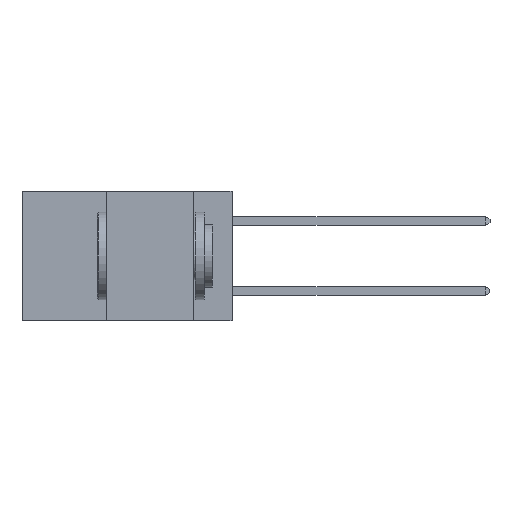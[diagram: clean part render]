
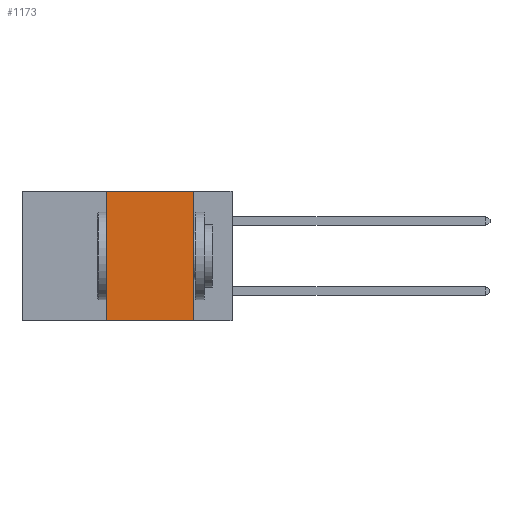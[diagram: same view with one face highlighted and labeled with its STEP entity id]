
A CAD part, left-side view. The second image highlights one B-rep face of the part: STEP entity #1173.
In plain terms, the highlighted planar face has unit normal (-1, 0, 0).
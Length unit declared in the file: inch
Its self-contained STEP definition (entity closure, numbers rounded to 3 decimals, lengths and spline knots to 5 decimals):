
#926 = DIRECTION ( 'NONE',  ( 0., -1., 0. ) ) ;
#1010 = CARTESIAN_POINT ( 'NONE',  ( 0., 0.6, -0.37 ) ) ;
#1046 = EDGE_LOOP ( 'NONE', ( #1762, #2713, #3122, #6306 ) ) ;
#1173 = ADVANCED_FACE ( 'NONE', ( #9684 ), #9001, .F. ) ;
#1283 = CARTESIAN_POINT ( 'NONE',  ( 0., 0.6, 0. ) ) ;
#1581 = VERTEX_POINT ( 'NONE', #3227 ) ;
#1762 = ORIENTED_EDGE ( 'NONE', *, *, #2248, .F. ) ;
#2248 = EDGE_CURVE ( 'NONE', #1581, #2544, #4500, .T. ) ;
#2544 = VERTEX_POINT ( 'NONE', #12754 ) ;
#2585 = DIRECTION ( 'NONE',  ( 0., 0., 1. ) ) ;
#2713 = ORIENTED_EDGE ( 'NONE', *, *, #12274, .F. ) ;
#2736 = AXIS2_PLACEMENT_3D ( 'NONE', #1283, #12302, #6659 ) ;
#3084 = CARTESIAN_POINT ( 'NONE',  ( 0., 0.36, 0. ) ) ;
#3122 = ORIENTED_EDGE ( 'NONE', *, *, #7905, .F. ) ;
#3227 = CARTESIAN_POINT ( 'NONE',  ( 0., 0.11, 0. ) ) ;
#3982 = EDGE_CURVE ( 'NONE', #7218, #2544, #7420, .T. ) ;
#4500 = LINE ( 'NONE', #4796, #7115 ) ;
#4545 = VECTOR ( 'NONE', #2585, 39.37008 ) ;
#4714 = DIRECTION ( 'NONE',  ( 0., 0., -1. ) ) ;
#4773 = CARTESIAN_POINT ( 'NONE',  ( 0., 0.36, -0.37 ) ) ;
#4796 = CARTESIAN_POINT ( 'NONE',  ( 0., 0.11, 0. ) ) ;
#4904 = LINE ( 'NONE', #9213, #4545 ) ;
#6137 = DIRECTION ( 'NONE',  ( 0., -1., 0. ) ) ;
#6235 = VERTEX_POINT ( 'NONE', #3084 ) ;
#6306 = ORIENTED_EDGE ( 'NONE', *, *, #3982, .T. ) ;
#6659 = DIRECTION ( 'NONE',  ( 0., 0., -1. ) ) ;
#6708 = VECTOR ( 'NONE', #926, 39.37008 ) ;
#7115 = VECTOR ( 'NONE', #4714, 39.37008 ) ;
#7218 = VERTEX_POINT ( 'NONE', #4773 ) ;
#7249 = CARTESIAN_POINT ( 'NONE',  ( 0., 0.6, 0. ) ) ;
#7420 = LINE ( 'NONE', #1010, #6708 ) ;
#7905 = EDGE_CURVE ( 'NONE', #7218, #6235, #4904, .T. ) ;
#9001 = PLANE ( 'NONE',  #2736 ) ;
#9213 = CARTESIAN_POINT ( 'NONE',  ( 0., 0.36, 0. ) ) ;
#9594 = LINE ( 'NONE', #7249, #11853 ) ;
#9684 = FACE_OUTER_BOUND ( 'NONE', #1046, .T. ) ;
#11853 = VECTOR ( 'NONE', #6137, 39.37008 ) ;
#12274 = EDGE_CURVE ( 'NONE', #6235, #1581, #9594, .T. ) ;
#12302 = DIRECTION ( 'NONE',  ( 1., 0., 0. ) ) ;
#12754 = CARTESIAN_POINT ( 'NONE',  ( 0., 0.11, -0.37 ) ) ;
